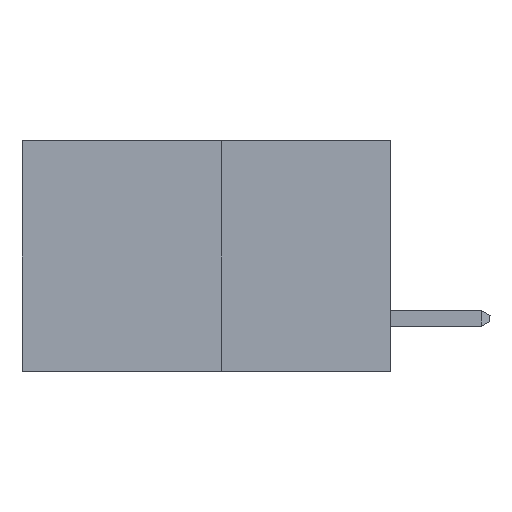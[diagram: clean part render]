
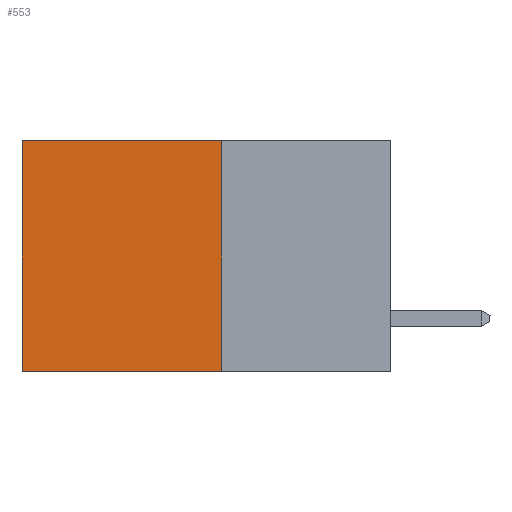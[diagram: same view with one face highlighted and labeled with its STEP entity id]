
A CAD part, left-side view. The second image highlights one B-rep face of the part: STEP entity #553.
In plain terms, the highlighted planar face has unit normal (-1, 0, 0).
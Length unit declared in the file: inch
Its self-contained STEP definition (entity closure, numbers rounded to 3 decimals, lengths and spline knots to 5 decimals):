
#195 = VERTEX_POINT ( 'NONE', #10517 ) ;
#383 = VECTOR ( 'NONE', #6790, 39.37008 ) ;
#553 = ADVANCED_FACE ( 'NONE', ( #1901 ), #9984, .F. ) ;
#578 = ORIENTED_EDGE ( 'NONE', *, *, #1580, .T. ) ;
#1310 = CARTESIAN_POINT ( 'NONE',  ( 0.277, 0.59, -0.37 ) ) ;
#1390 = ORIENTED_EDGE ( 'NONE', *, *, #10223, .T. ) ;
#1580 = EDGE_CURVE ( 'NONE', #4262, #2651, #5096, .T. ) ;
#1597 = EDGE_CURVE ( 'NONE', #195, #2651, #2453, .T. ) ;
#1807 = DIRECTION ( 'NONE',  ( 0., 0., -1. ) ) ;
#1901 = FACE_OUTER_BOUND ( 'NONE', #4484, .T. ) ;
#2134 = VERTEX_POINT ( 'NONE', #6226 ) ;
#2318 = CARTESIAN_POINT ( 'NONE',  ( 0.277, 0.59, -0.37 ) ) ;
#2453 = LINE ( 'NONE', #7883, #383 ) ;
#2651 = VERTEX_POINT ( 'NONE', #2318 ) ;
#2727 = VECTOR ( 'NONE', #1807, 39.37008 ) ;
#2988 = DIRECTION ( 'NONE',  ( 0., 0., -1. ) ) ;
#3218 = ORIENTED_EDGE ( 'NONE', *, *, #8350, .F. ) ;
#3613 = VECTOR ( 'NONE', #7503, 39.37008 ) ;
#4262 = VERTEX_POINT ( 'NONE', #9191 ) ;
#4408 = CARTESIAN_POINT ( 'NONE',  ( 0.277, 0.27, -0.37 ) ) ;
#4462 = LINE ( 'NONE', #5800, #3613 ) ;
#4484 = EDGE_LOOP ( 'NONE', ( #578, #9662, #3218, #1390 ) ) ;
#5096 = LINE ( 'NONE', #1310, #2727 ) ;
#5372 = CARTESIAN_POINT ( 'NONE',  ( 0.277, 0.27, -0.37 ) ) ;
#5800 = CARTESIAN_POINT ( 'NONE',  ( 0.277, 0.27, 0. ) ) ;
#6226 = CARTESIAN_POINT ( 'NONE',  ( 0.277, 0.27, 0. ) ) ;
#6236 = DIRECTION ( 'NONE',  ( 0., 0., -1. ) ) ;
#6384 = LINE ( 'NONE', #5372, #10456 ) ;
#6790 = DIRECTION ( 'NONE',  ( 0., 1., 0. ) ) ;
#7503 = DIRECTION ( 'NONE',  ( 0., 1., 0. ) ) ;
#7883 = CARTESIAN_POINT ( 'NONE',  ( 0.277, 0.27, -0.37 ) ) ;
#8029 = AXIS2_PLACEMENT_3D ( 'NONE', #4408, #10588, #2988 ) ;
#8350 = EDGE_CURVE ( 'NONE', #2134, #195, #6384, .T. ) ;
#9191 = CARTESIAN_POINT ( 'NONE',  ( 0.277, 0.59, 0. ) ) ;
#9662 = ORIENTED_EDGE ( 'NONE', *, *, #1597, .F. ) ;
#9984 = PLANE ( 'NONE',  #8029 ) ;
#10223 = EDGE_CURVE ( 'NONE', #2134, #4262, #4462, .T. ) ;
#10456 = VECTOR ( 'NONE', #6236, 39.37008 ) ;
#10517 = CARTESIAN_POINT ( 'NONE',  ( 0.277, 0.27, -0.37 ) ) ;
#10588 = DIRECTION ( 'NONE',  ( 1., 0., 0. ) ) ;
